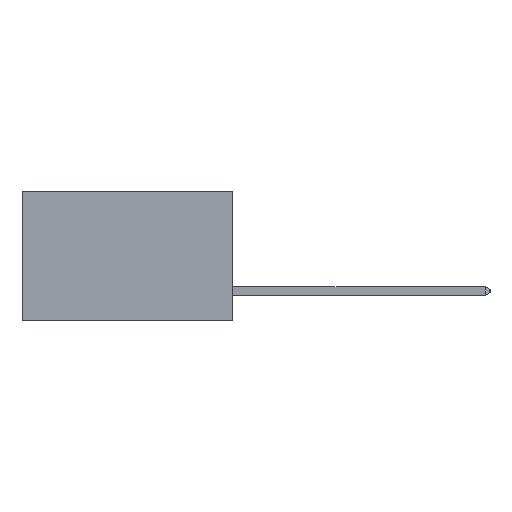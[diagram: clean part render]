
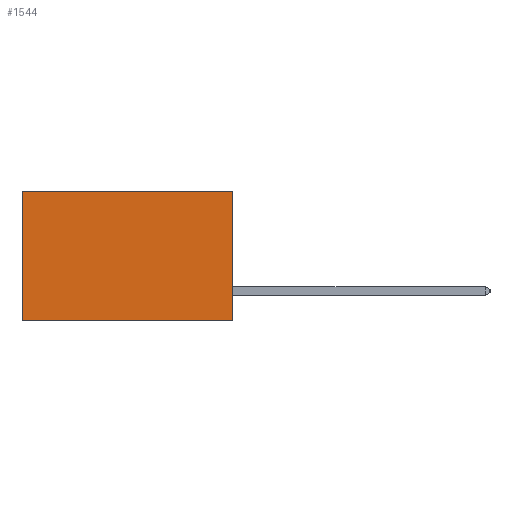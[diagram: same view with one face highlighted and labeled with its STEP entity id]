
A CAD part, left-side view. The second image highlights one B-rep face of the part: STEP entity #1544.
In plain terms, the highlighted planar face has unit normal (-1, 0, 0).
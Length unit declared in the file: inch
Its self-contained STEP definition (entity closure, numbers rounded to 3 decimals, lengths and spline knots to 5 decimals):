
#1544 = ADVANCED_FACE ( 'NONE', ( #16043 ), #4147, .F. ) ;
#3140 = ORIENTED_EDGE ( 'NONE', *, *, #26473, .F. ) ;
#3456 = VECTOR ( 'NONE', #7884, 39.37008 ) ;
#3968 = VERTEX_POINT ( 'NONE', #4742 ) ;
#4147 = PLANE ( 'NONE',  #8088 ) ;
#4436 = CARTESIAN_POINT ( 'NONE',  ( 0.2875, 0., 0. ) ) ;
#4742 = CARTESIAN_POINT ( 'NONE',  ( 0.2875, 0., 0. ) ) ;
#4882 = CARTESIAN_POINT ( 'NONE',  ( 0.2875, 0., 0. ) ) ;
#5062 = EDGE_CURVE ( 'NONE', #25558, #24289, #24116, .T. ) ;
#6643 = EDGE_CURVE ( 'NONE', #3968, #19452, #8074, .T. ) ;
#6701 = CARTESIAN_POINT ( 'NONE',  ( 0.2875, 0., -0.37 ) ) ;
#6986 = DIRECTION ( 'NONE',  ( 0., 1., 0. ) ) ;
#7570 = DIRECTION ( 'NONE',  ( 0., 0., -1. ) ) ;
#7884 = DIRECTION ( 'NONE',  ( 0., 1., 0. ) ) ;
#8074 = LINE ( 'NONE', #4882, #23791 ) ;
#8076 = LINE ( 'NONE', #17872, #8752 ) ;
#8088 = AXIS2_PLACEMENT_3D ( 'NONE', #4436, #20874, #8184 ) ;
#8184 = DIRECTION ( 'NONE',  ( 0., 0., -1. ) ) ;
#8752 = VECTOR ( 'NONE', #7570, 39.37008 ) ;
#11210 = EDGE_LOOP ( 'NONE', ( #23718, #25127, #3140, #26364 ) ) ;
#12033 = LINE ( 'NONE', #26318, #17451 ) ;
#13574 = CARTESIAN_POINT ( 'NONE',  ( 0.2875, 0.6, -0.37 ) ) ;
#14276 = DIRECTION ( 'NONE',  ( 0., 0., -1. ) ) ;
#16043 = FACE_OUTER_BOUND ( 'NONE', #11210, .T. ) ;
#17451 = VECTOR ( 'NONE', #14276, 39.37008 ) ;
#17822 = EDGE_CURVE ( 'NONE', #19452, #24289, #12033, .T. ) ;
#17872 = CARTESIAN_POINT ( 'NONE',  ( 0.2875, 0., 0. ) ) ;
#19452 = VERTEX_POINT ( 'NONE', #22933 ) ;
#20874 = DIRECTION ( 'NONE',  ( 1., 0., 0. ) ) ;
#22269 = CARTESIAN_POINT ( 'NONE',  ( 0.2875, 0., -0.37 ) ) ;
#22933 = CARTESIAN_POINT ( 'NONE',  ( 0.2875, 0.6, 0. ) ) ;
#23718 = ORIENTED_EDGE ( 'NONE', *, *, #17822, .T. ) ;
#23791 = VECTOR ( 'NONE', #6986, 39.37008 ) ;
#24116 = LINE ( 'NONE', #22269, #3456 ) ;
#24289 = VERTEX_POINT ( 'NONE', #13574 ) ;
#25127 = ORIENTED_EDGE ( 'NONE', *, *, #5062, .F. ) ;
#25558 = VERTEX_POINT ( 'NONE', #6701 ) ;
#26318 = CARTESIAN_POINT ( 'NONE',  ( 0.2875, 0.6, 0. ) ) ;
#26364 = ORIENTED_EDGE ( 'NONE', *, *, #6643, .T. ) ;
#26473 = EDGE_CURVE ( 'NONE', #3968, #25558, #8076, .T. ) ;
